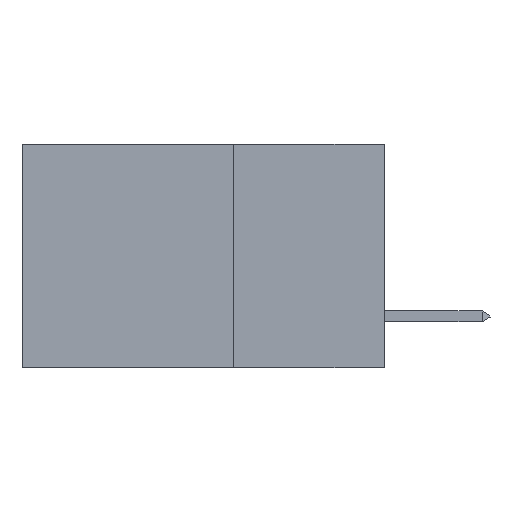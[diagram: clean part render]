
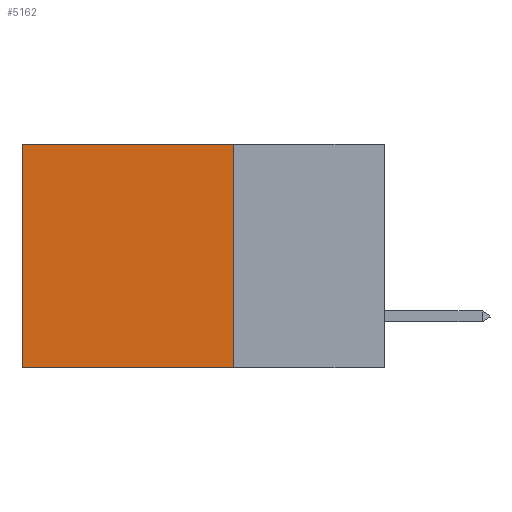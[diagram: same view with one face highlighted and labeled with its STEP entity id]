
A CAD part, left-side view. The second image highlights one B-rep face of the part: STEP entity #5162.
In plain terms, the highlighted planar face has unit normal (-1, 0, 0).
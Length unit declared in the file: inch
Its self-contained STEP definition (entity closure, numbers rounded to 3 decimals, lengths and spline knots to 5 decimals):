
#68 = DIRECTION ( 'NONE',  ( 1., 0., 0. ) ) ;
#370 = VECTOR ( 'NONE', #6894, 39.37008 ) ;
#664 = FACE_OUTER_BOUND ( 'NONE', #5456, .T. ) ;
#843 = DIRECTION ( 'NONE',  ( 0., 0., -1. ) ) ;
#1034 = EDGE_CURVE ( 'NONE', #3098, #6443, #1201, .T. ) ;
#1201 = LINE ( 'NONE', #2785, #5267 ) ;
#1328 = DIRECTION ( 'NONE',  ( 0., 1., 0. ) ) ;
#1387 = LINE ( 'NONE', #6969, #3897 ) ;
#1979 = VERTEX_POINT ( 'NONE', #4481 ) ;
#2229 = CARTESIAN_POINT ( 'NONE',  ( 0.2875, 0.25, -0.37 ) ) ;
#2785 = CARTESIAN_POINT ( 'NONE',  ( 0.2875, 0.25, 0. ) ) ;
#2827 = PLANE ( 'NONE',  #2853 ) ;
#2853 = AXIS2_PLACEMENT_3D ( 'NONE', #10969, #68, #4645 ) ;
#3098 = VERTEX_POINT ( 'NONE', #8502 ) ;
#3153 = ORIENTED_EDGE ( 'NONE', *, *, #1034, .F. ) ;
#3833 = ORIENTED_EDGE ( 'NONE', *, *, #7379, .T. ) ;
#3897 = VECTOR ( 'NONE', #7086, 39.37008 ) ;
#4481 = CARTESIAN_POINT ( 'NONE',  ( 0.2875, 0.6, 0. ) ) ;
#4645 = DIRECTION ( 'NONE',  ( 0., 0., -1. ) ) ;
#4721 = CARTESIAN_POINT ( 'NONE',  ( 0.2875, 0.6, -0.37 ) ) ;
#5162 = ADVANCED_FACE ( 'NONE', ( #664 ), #2827, .F. ) ;
#5253 = VECTOR ( 'NONE', #1328, 39.37008 ) ;
#5267 = VECTOR ( 'NONE', #843, 39.37008 ) ;
#5456 = EDGE_LOOP ( 'NONE', ( #3833, #10634, #3153, #10610 ) ) ;
#5535 = CARTESIAN_POINT ( 'NONE',  ( 0.2875, 0.25, -0.37 ) ) ;
#6443 = VERTEX_POINT ( 'NONE', #5535 ) ;
#6894 = DIRECTION ( 'NONE',  ( 0., 1., 0. ) ) ;
#6969 = CARTESIAN_POINT ( 'NONE',  ( 0.2875, 0.6, 0. ) ) ;
#7086 = DIRECTION ( 'NONE',  ( 0., 0., -1. ) ) ;
#7379 = EDGE_CURVE ( 'NONE', #1979, #10915, #1387, .T. ) ;
#7900 = CARTESIAN_POINT ( 'NONE',  ( 0.2875, 0.25, 0. ) ) ;
#8502 = CARTESIAN_POINT ( 'NONE',  ( 0.2875, 0.25, 0. ) ) ;
#8544 = EDGE_CURVE ( 'NONE', #3098, #1979, #11317, .T. ) ;
#9430 = LINE ( 'NONE', #2229, #5253 ) ;
#9739 = EDGE_CURVE ( 'NONE', #6443, #10915, #9430, .T. ) ;
#10610 = ORIENTED_EDGE ( 'NONE', *, *, #8544, .T. ) ;
#10634 = ORIENTED_EDGE ( 'NONE', *, *, #9739, .F. ) ;
#10915 = VERTEX_POINT ( 'NONE', #4721 ) ;
#10969 = CARTESIAN_POINT ( 'NONE',  ( 0.2875, 0.25, 0. ) ) ;
#11317 = LINE ( 'NONE', #7900, #370 ) ;
